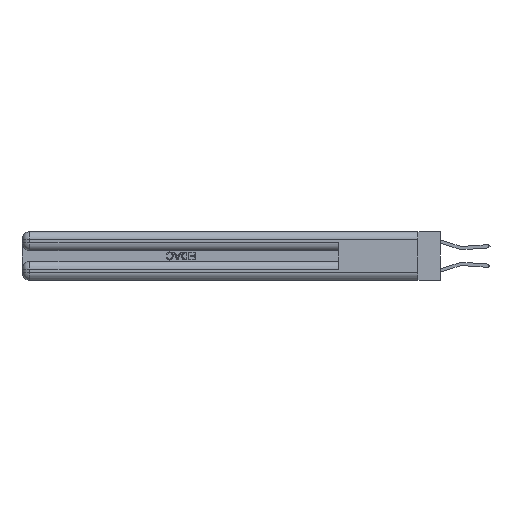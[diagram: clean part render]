
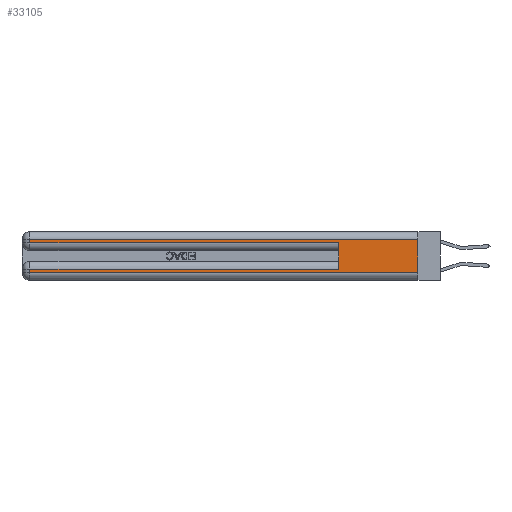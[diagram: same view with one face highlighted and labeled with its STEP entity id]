
A CAD part, left-side view. The second image highlights one B-rep face of the part: STEP entity #33105.
In plain terms, the highlighted planar face has unit normal (-1, 0, 0).
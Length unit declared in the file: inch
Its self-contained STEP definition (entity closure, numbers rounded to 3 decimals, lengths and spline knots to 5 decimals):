
#876 = LINE ( 'NONE', #11422, #3768 ) ;
#1689 = DIRECTION ( 'NONE',  ( 0., -1., 0. ) ) ;
#1823 = CARTESIAN_POINT ( 'NONE',  ( 0., 0.6, 0.085 ) ) ;
#2697 = VECTOR ( 'NONE', #23119, 39.37008 ) ;
#3078 = ORIENTED_EDGE ( 'NONE', *, *, #4601, .F. ) ;
#3184 = PLANE ( 'NONE',  #11322 ) ;
#3288 = EDGE_CURVE ( 'NONE', #9742, #24548, #9399, .T. ) ;
#3762 = EDGE_CURVE ( 'NONE', #25874, #30955, #14740, .T. ) ;
#3768 = VECTOR ( 'NONE', #28513, 39.37008 ) ;
#3993 = CARTESIAN_POINT ( 'NONE',  ( 0., 0.6, 0.285 ) ) ;
#4601 = EDGE_CURVE ( 'NONE', #19174, #27812, #4893, .T. ) ;
#4857 = LINE ( 'NONE', #33029, #19207 ) ;
#4893 = LINE ( 'NONE', #12271, #34409 ) ;
#5113 = EDGE_CURVE ( 'NONE', #19174, #25874, #12445, .T. ) ;
#5653 = CARTESIAN_POINT ( 'NONE',  ( 0., 2.94, 0.085 ) ) ;
#6052 = CARTESIAN_POINT ( 'NONE',  ( 0., 0., 0.37 ) ) ;
#8927 = DIRECTION ( 'NONE',  ( 0., 0., -1. ) ) ;
#9075 = CARTESIAN_POINT ( 'NONE',  ( 0., 0., 0.06 ) ) ;
#9399 = LINE ( 'NONE', #20139, #2697 ) ;
#9623 = ORIENTED_EDGE ( 'NONE', *, *, #15259, .T. ) ;
#9742 = VERTEX_POINT ( 'NONE', #1823 ) ;
#10850 = CARTESIAN_POINT ( 'NONE',  ( 0., 2.94, 0.37 ) ) ;
#11322 = AXIS2_PLACEMENT_3D ( 'NONE', #6052, #26038, #8927 ) ;
#11422 = CARTESIAN_POINT ( 'NONE',  ( 0., 0.6, 0.145 ) ) ;
#11450 = CARTESIAN_POINT ( 'NONE',  ( 0., 2.94, 0.37 ) ) ;
#11506 = DIRECTION ( 'NONE',  ( 0., 1., 0. ) ) ;
#11545 = LINE ( 'NONE', #18859, #33456 ) ;
#11570 = DIRECTION ( 'NONE',  ( 0., 0., -1. ) ) ;
#12271 = CARTESIAN_POINT ( 'NONE',  ( 0., 0., 0.37 ) ) ;
#12445 = LINE ( 'NONE', #31498, #33475 ) ;
#13281 = VERTEX_POINT ( 'NONE', #3993 ) ;
#14740 = LINE ( 'NONE', #10850, #29468 ) ;
#15259 = EDGE_CURVE ( 'NONE', #27718, #27812, #4857, .T. ) ;
#16550 = EDGE_CURVE ( 'NONE', #30955, #13281, #11545, .T. ) ;
#17234 = CARTESIAN_POINT ( 'NONE',  ( 0., 2.94, 0.31 ) ) ;
#18859 = CARTESIAN_POINT ( 'NONE',  ( 0., 0., 0.285 ) ) ;
#19174 = VERTEX_POINT ( 'NONE', #31894 ) ;
#19207 = VECTOR ( 'NONE', #35898, 39.37008 ) ;
#20139 = CARTESIAN_POINT ( 'NONE',  ( 0., 0., 0.085 ) ) ;
#21923 = ORIENTED_EDGE ( 'NONE', *, *, #16550, .T. ) ;
#22918 = ORIENTED_EDGE ( 'NONE', *, *, #24542, .F. ) ;
#23119 = DIRECTION ( 'NONE',  ( 0., 1., 0. ) ) ;
#23846 = ORIENTED_EDGE ( 'NONE', *, *, #35054, .T. ) ;
#24542 = EDGE_CURVE ( 'NONE', #9742, #13281, #876, .T. ) ;
#24548 = VERTEX_POINT ( 'NONE', #5653 ) ;
#25874 = VERTEX_POINT ( 'NONE', #17234 ) ;
#26038 = DIRECTION ( 'NONE',  ( 1., 0., 0. ) ) ;
#26181 = VECTOR ( 'NONE', #11570, 39.37008 ) ;
#26504 = DIRECTION ( 'NONE',  ( 0., 0., -1. ) ) ;
#26698 = CARTESIAN_POINT ( 'NONE',  ( 0., 2.94, 0.285 ) ) ;
#27718 = VERTEX_POINT ( 'NONE', #31334 ) ;
#27812 = VERTEX_POINT ( 'NONE', #9075 ) ;
#27962 = LINE ( 'NONE', #11450, #26181 ) ;
#28513 = DIRECTION ( 'NONE',  ( 0., 0., 1. ) ) ;
#29468 = VECTOR ( 'NONE', #33706, 39.37008 ) ;
#30458 = ORIENTED_EDGE ( 'NONE', *, *, #3288, .T. ) ;
#30955 = VERTEX_POINT ( 'NONE', #26698 ) ;
#31237 = EDGE_LOOP ( 'NONE', ( #3078, #36530, #33269, #21923, #22918, #30458, #23846, #9623 ) ) ;
#31334 = CARTESIAN_POINT ( 'NONE',  ( 0., 2.94, 0.06 ) ) ;
#31498 = CARTESIAN_POINT ( 'NONE',  ( 0., 0., 0.31 ) ) ;
#31894 = CARTESIAN_POINT ( 'NONE',  ( 0., 0., 0.31 ) ) ;
#33029 = CARTESIAN_POINT ( 'NONE',  ( 0., 0., 0.06 ) ) ;
#33105 = ADVANCED_FACE ( 'NONE', ( #36106 ), #3184, .F. ) ;
#33269 = ORIENTED_EDGE ( 'NONE', *, *, #3762, .T. ) ;
#33456 = VECTOR ( 'NONE', #1689, 39.37008 ) ;
#33475 = VECTOR ( 'NONE', #11506, 39.37008 ) ;
#33706 = DIRECTION ( 'NONE',  ( 0., 0., -1. ) ) ;
#34409 = VECTOR ( 'NONE', #26504, 39.37008 ) ;
#35054 = EDGE_CURVE ( 'NONE', #24548, #27718, #27962, .T. ) ;
#35898 = DIRECTION ( 'NONE',  ( 0., -1., 0. ) ) ;
#36106 = FACE_OUTER_BOUND ( 'NONE', #31237, .T. ) ;
#36530 = ORIENTED_EDGE ( 'NONE', *, *, #5113, .T. ) ;
